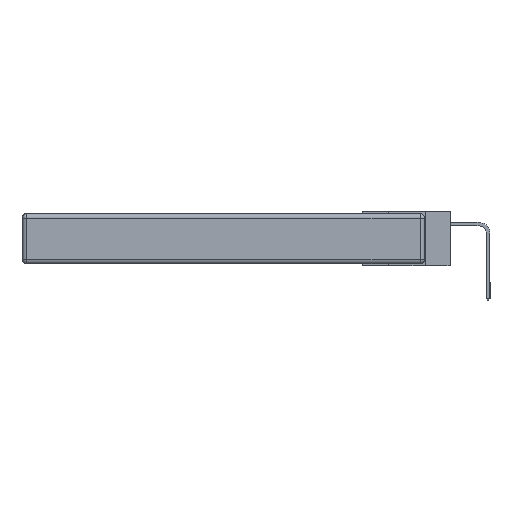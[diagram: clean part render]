
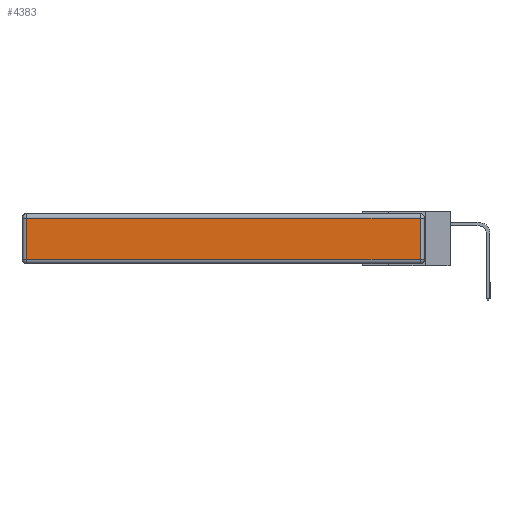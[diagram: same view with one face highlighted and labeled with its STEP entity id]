
A CAD part, left-side view. The second image highlights one B-rep face of the part: STEP entity #4383.
In plain terms, the highlighted planar face has unit normal (-1, 0, 0).
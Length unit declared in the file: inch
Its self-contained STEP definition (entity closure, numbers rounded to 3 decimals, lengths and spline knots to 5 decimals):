
#85 = ORIENTED_EDGE ( 'NONE', *, *, #7855, .T. ) ;
#474 = VECTOR ( 'NONE', #25467, 39.37008 ) ;
#855 = CARTESIAN_POINT ( 'NONE',  ( 0., 2.72, -0.03 ) ) ;
#3211 = DIRECTION ( 'NONE',  ( 0., 0., -1. ) ) ;
#3296 = CARTESIAN_POINT ( 'NONE',  ( 0., 2.72, -0.343 ) ) ;
#3967 = LINE ( 'NONE', #3296, #6886 ) ;
#4129 = EDGE_CURVE ( 'NONE', #20414, #11302, #20990, .T. ) ;
#4383 = ADVANCED_FACE ( 'NONE', ( #6798 ), #10341, .T. ) ;
#5241 = EDGE_CURVE ( 'NONE', #11302, #26501, #11467, .T. ) ;
#6798 = FACE_OUTER_BOUND ( 'NONE', #22968, .T. ) ;
#6886 = VECTOR ( 'NONE', #3211, 39.37008 ) ;
#7855 = EDGE_CURVE ( 'NONE', #26553, #20414, #22664, .T. ) ;
#8410 = AXIS2_PLACEMENT_3D ( 'NONE', #22911, #12581, #21797 ) ;
#9184 = ORIENTED_EDGE ( 'NONE', *, *, #5241, .T. ) ;
#10341 = PLANE ( 'NONE',  #8410 ) ;
#10822 = CARTESIAN_POINT ( 'NONE',  ( 0., 2.72, -0.313 ) ) ;
#10877 = CARTESIAN_POINT ( 'NONE',  ( 0., 0.03, -0.343 ) ) ;
#11302 = VERTEX_POINT ( 'NONE', #23115 ) ;
#11467 = LINE ( 'NONE', #17353, #474 ) ;
#11499 = CARTESIAN_POINT ( 'NONE',  ( 0., 0.03, -0.313 ) ) ;
#12581 = DIRECTION ( 'NONE',  ( -1., 0., 0. ) ) ;
#13917 = DIRECTION ( 'NONE',  ( 0., -1., 0. ) ) ;
#16371 = ORIENTED_EDGE ( 'NONE', *, *, #19272, .T. ) ;
#17103 = VECTOR ( 'NONE', #25187, 39.37008 ) ;
#17353 = CARTESIAN_POINT ( 'NONE',  ( 0., 2.75, -0.03 ) ) ;
#19272 = EDGE_CURVE ( 'NONE', #26501, #26553, #3967, .T. ) ;
#20414 = VERTEX_POINT ( 'NONE', #11499 ) ;
#20990 = LINE ( 'NONE', #10877, #17103 ) ;
#21778 = ORIENTED_EDGE ( 'NONE', *, *, #4129, .T. ) ;
#21797 = DIRECTION ( 'NONE',  ( 0., 0., 1. ) ) ;
#22176 = CARTESIAN_POINT ( 'NONE',  ( 0., 0., -0.313 ) ) ;
#22664 = LINE ( 'NONE', #22176, #24954 ) ;
#22911 = CARTESIAN_POINT ( 'NONE',  ( 0., 0., -0.343 ) ) ;
#22968 = EDGE_LOOP ( 'NONE', ( #85, #21778, #9184, #16371 ) ) ;
#23115 = CARTESIAN_POINT ( 'NONE',  ( 0., 0.03, -0.03 ) ) ;
#24954 = VECTOR ( 'NONE', #13917, 39.37008 ) ;
#25187 = DIRECTION ( 'NONE',  ( 0., 0., 1. ) ) ;
#25467 = DIRECTION ( 'NONE',  ( 0., 1., 0. ) ) ;
#26501 = VERTEX_POINT ( 'NONE', #855 ) ;
#26553 = VERTEX_POINT ( 'NONE', #10822 ) ;
